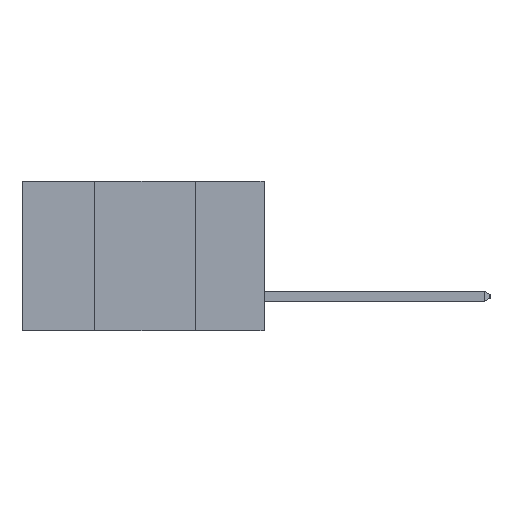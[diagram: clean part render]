
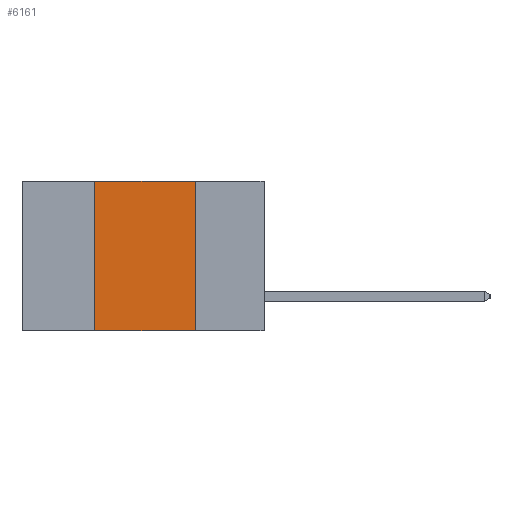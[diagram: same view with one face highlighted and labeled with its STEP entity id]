
A CAD part, left-side view. The second image highlights one B-rep face of the part: STEP entity #6161.
In plain terms, the highlighted planar face has unit normal (-1, 0, 0).
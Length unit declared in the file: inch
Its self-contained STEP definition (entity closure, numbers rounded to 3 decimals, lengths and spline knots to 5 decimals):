
#252 = VERTEX_POINT ( 'NONE', #1124 ) ;
#280 = VECTOR ( 'NONE', #2326, 39.37008 ) ;
#433 = CARTESIAN_POINT ( 'NONE',  ( 0., 0.17, -0.37 ) ) ;
#534 = CARTESIAN_POINT ( 'NONE',  ( 0., 0.17, -0.37 ) ) ;
#761 = FACE_OUTER_BOUND ( 'NONE', #6159, .T. ) ;
#987 = CARTESIAN_POINT ( 'NONE',  ( 0., 0.42, -0.37 ) ) ;
#1124 = CARTESIAN_POINT ( 'NONE',  ( 0., 0.42, -0.37 ) ) ;
#1233 = VECTOR ( 'NONE', #11323, 39.37008 ) ;
#1591 = LINE ( 'NONE', #8677, #1233 ) ;
#1639 = CARTESIAN_POINT ( 'NONE',  ( 0., 0.6, 0. ) ) ;
#2063 = EDGE_CURVE ( 'NONE', #252, #7871, #11020, .T. ) ;
#2326 = DIRECTION ( 'NONE',  ( 0., 0., 1. ) ) ;
#2359 = VECTOR ( 'NONE', #8899, 39.37008 ) ;
#2743 = PLANE ( 'NONE',  #7387 ) ;
#4140 = VECTOR ( 'NONE', #11486, 39.37008 ) ;
#5013 = DIRECTION ( 'NONE',  ( 0., 0., -1. ) ) ;
#5227 = ORIENTED_EDGE ( 'NONE', *, *, #11210, .T. ) ;
#5893 = DIRECTION ( 'NONE',  ( 1., 0., 0. ) ) ;
#5932 = CARTESIAN_POINT ( 'NONE',  ( 0., 0.6, 0. ) ) ;
#6159 = EDGE_LOOP ( 'NONE', ( #10758, #6714, #7924, #5227 ) ) ;
#6161 = ADVANCED_FACE ( 'NONE', ( #761 ), #2743, .F. ) ;
#6714 = ORIENTED_EDGE ( 'NONE', *, *, #12144, .F. ) ;
#6816 = LINE ( 'NONE', #1639, #4140 ) ;
#7387 = AXIS2_PLACEMENT_3D ( 'NONE', #5932, #5893, #5013 ) ;
#7871 = VERTEX_POINT ( 'NONE', #10910 ) ;
#7924 = ORIENTED_EDGE ( 'NONE', *, *, #2063, .F. ) ;
#8677 = CARTESIAN_POINT ( 'NONE',  ( 0., 0.6, -0.37 ) ) ;
#8899 = DIRECTION ( 'NONE',  ( 0., 0., -1. ) ) ;
#9592 = VERTEX_POINT ( 'NONE', #433 ) ;
#9626 = VERTEX_POINT ( 'NONE', #12308 ) ;
#9670 = EDGE_CURVE ( 'NONE', #9626, #9592, #10247, .T. ) ;
#10247 = LINE ( 'NONE', #534, #2359 ) ;
#10758 = ORIENTED_EDGE ( 'NONE', *, *, #9670, .F. ) ;
#10910 = CARTESIAN_POINT ( 'NONE',  ( 0., 0.42, 0. ) ) ;
#11020 = LINE ( 'NONE', #987, #280 ) ;
#11210 = EDGE_CURVE ( 'NONE', #252, #9592, #1591, .T. ) ;
#11323 = DIRECTION ( 'NONE',  ( 0., -1., 0. ) ) ;
#11486 = DIRECTION ( 'NONE',  ( 0., -1., 0. ) ) ;
#12144 = EDGE_CURVE ( 'NONE', #7871, #9626, #6816, .T. ) ;
#12308 = CARTESIAN_POINT ( 'NONE',  ( 0., 0.17, 0. ) ) ;
